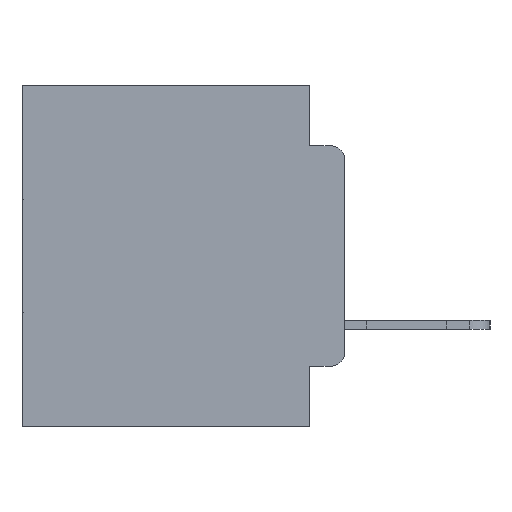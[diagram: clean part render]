
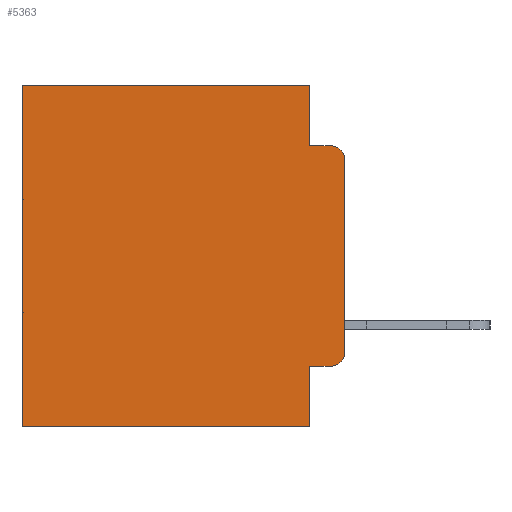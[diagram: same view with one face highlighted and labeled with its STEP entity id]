
A CAD part, left-side view. The second image highlights one B-rep face of the part: STEP entity #5363.
In plain terms, the highlighted planar face has unit normal (-1, 0, 0).
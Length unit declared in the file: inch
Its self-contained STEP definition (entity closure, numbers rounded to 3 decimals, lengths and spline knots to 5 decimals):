
#291 = EDGE_CURVE ( 'NONE', #7167, #15335, #7484, .T. ) ;
#449 = VERTEX_POINT ( 'NONE', #22604 ) ;
#1073 = VERTEX_POINT ( 'NONE', #19541 ) ;
#1476 = VERTEX_POINT ( 'NONE', #2860 ) ;
#1525 = DIRECTION ( 'NONE',  ( -1., 0., 0. ) ) ;
#1810 = ORIENTED_EDGE ( 'NONE', *, *, #14209, .T. ) ;
#1933 = VECTOR ( 'NONE', #9088, 39.37008 ) ;
#2264 = CARTESIAN_POINT ( 'NONE',  ( 0.298, 0.051, 0. ) ) ;
#2412 = ORIENTED_EDGE ( 'NONE', *, *, #7960, .T. ) ;
#2860 = CARTESIAN_POINT ( 'NONE',  ( 0.298, 0.473, -0.5 ) ) ;
#3824 = VERTEX_POINT ( 'NONE', #19217 ) ;
#3989 = CARTESIAN_POINT ( 'NONE',  ( 0.298, 0., 0. ) ) ;
#4005 = DIRECTION ( 'NONE',  ( 0., -1., 0. ) ) ;
#4414 = CARTESIAN_POINT ( 'NONE',  ( 0.298, 0., -0.5 ) ) ;
#4771 = FACE_OUTER_BOUND ( 'NONE', #26097, .T. ) ;
#5363 = ADVANCED_FACE ( 'NONE', ( #4771 ), #12246, .F. ) ;
#6403 = EDGE_CURVE ( 'NONE', #25711, #7167, #6469, .T. ) ;
#6469 = LINE ( 'NONE', #2264, #18177 ) ;
#7167 = VERTEX_POINT ( 'NONE', #20082 ) ;
#7484 = LINE ( 'NONE', #11281, #19053 ) ;
#7605 = VERTEX_POINT ( 'NONE', #22730 ) ;
#7831 = DIRECTION ( 'NONE',  ( 0., 0., -1. ) ) ;
#7960 = EDGE_CURVE ( 'NONE', #3824, #15335, #20650, .T. ) ;
#8324 = ORIENTED_EDGE ( 'NONE', *, *, #10698, .T. ) ;
#8485 = EDGE_CURVE ( 'NONE', #1073, #1476, #8627, .T. ) ;
#8627 = LINE ( 'NONE', #4414, #1933 ) ;
#8784 = VERTEX_POINT ( 'NONE', #15536 ) ;
#8816 = ORIENTED_EDGE ( 'NONE', *, *, #9880, .T. ) ;
#9088 = DIRECTION ( 'NONE',  ( 0., 1., 0. ) ) ;
#9880 = EDGE_CURVE ( 'NONE', #25711, #8784, #24725, .T. ) ;
#10514 = DIRECTION ( 'NONE',  ( 0., 1., 0. ) ) ;
#10698 = EDGE_CURVE ( 'NONE', #8784, #1476, #17287, .T. ) ;
#11136 = AXIS2_PLACEMENT_3D ( 'NONE', #26998, #1525, #18008 ) ;
#11281 = CARTESIAN_POINT ( 'NONE',  ( 0.298, 0.051, -0.0885 ) ) ;
#11382 = CARTESIAN_POINT ( 'NONE',  ( 0.298, 0.051, 0. ) ) ;
#11774 = ORIENTED_EDGE ( 'NONE', *, *, #6403, .F. ) ;
#11890 = VECTOR ( 'NONE', #7831, 39.37008 ) ;
#12166 = VECTOR ( 'NONE', #25401, 39.37008 ) ;
#12246 = PLANE ( 'NONE',  #12442 ) ;
#12442 = AXIS2_PLACEMENT_3D ( 'NONE', #13769, #15332, #23437 ) ;
#13073 = VECTOR ( 'NONE', #10514, 39.37008 ) ;
#13224 = DIRECTION ( 'NONE',  ( 0., 0., -1. ) ) ;
#13307 = LINE ( 'NONE', #29757, #24258 ) ;
#13460 = DIRECTION ( 'NONE',  ( 0., -1., 0. ) ) ;
#13769 = CARTESIAN_POINT ( 'NONE',  ( 0.298, 0., 0. ) ) ;
#13771 = DIRECTION ( 'NONE',  ( 0., 0., -1. ) ) ;
#14209 = EDGE_CURVE ( 'NONE', #449, #29352, #13307, .T. ) ;
#14313 = ORIENTED_EDGE ( 'NONE', *, *, #23508, .F. ) ;
#15332 = DIRECTION ( 'NONE',  ( 1., 0., 0. ) ) ;
#15335 = VERTEX_POINT ( 'NONE', #17015 ) ;
#15450 = ORIENTED_EDGE ( 'NONE', *, *, #291, .F. ) ;
#15484 = ORIENTED_EDGE ( 'NONE', *, *, #28410, .F. ) ;
#15513 = CARTESIAN_POINT ( 'NONE',  ( 0.298, 0.051, 0. ) ) ;
#15536 = CARTESIAN_POINT ( 'NONE',  ( 0.298, 0.473, 0. ) ) ;
#15918 = CARTESIAN_POINT ( 'NONE',  ( 0.298, 0.02, -0.1085 ) ) ;
#16271 = DIRECTION ( 'NONE',  ( 0., 0., -1. ) ) ;
#17015 = CARTESIAN_POINT ( 'NONE',  ( 0.298, 0.02, -0.0885 ) ) ;
#17287 = LINE ( 'NONE', #19872, #11890 ) ;
#18008 = DIRECTION ( 'NONE',  ( 0., 0., -1. ) ) ;
#18177 = VECTOR ( 'NONE', #16271, 39.37008 ) ;
#18669 = CARTESIAN_POINT ( 'NONE',  ( 0.298, 0.02, -0.4115 ) ) ;
#18683 = ORIENTED_EDGE ( 'NONE', *, *, #29575, .T. ) ;
#19053 = VECTOR ( 'NONE', #13460, 39.37008 ) ;
#19217 = CARTESIAN_POINT ( 'NONE',  ( 0.298, 0., -0.1085 ) ) ;
#19541 = CARTESIAN_POINT ( 'NONE',  ( 0.298, 0.051, -0.5 ) ) ;
#19795 = ORIENTED_EDGE ( 'NONE', *, *, #8485, .F. ) ;
#19872 = CARTESIAN_POINT ( 'NONE',  ( 0.298, 0.473, 0. ) ) ;
#20082 = CARTESIAN_POINT ( 'NONE',  ( 0.298, 0.051, -0.0885 ) ) ;
#20650 = CIRCLE ( 'NONE', #24309, 0.02 ) ;
#22604 = CARTESIAN_POINT ( 'NONE',  ( 0.298, 0.051, -0.4115 ) ) ;
#22730 = CARTESIAN_POINT ( 'NONE',  ( 0.298, 0., -0.3915 ) ) ;
#23437 = DIRECTION ( 'NONE',  ( 0., 0., -1. ) ) ;
#23508 = EDGE_CURVE ( 'NONE', #449, #1073, #24585, .T. ) ;
#23892 = VECTOR ( 'NONE', #13224, 39.37008 ) ;
#24258 = VECTOR ( 'NONE', #4005, 39.37008 ) ;
#24309 = AXIS2_PLACEMENT_3D ( 'NONE', #15918, #28979, #13771 ) ;
#24585 = LINE ( 'NONE', #11382, #23892 ) ;
#24590 = LINE ( 'NONE', #3989, #12166 ) ;
#24725 = LINE ( 'NONE', #24901, #13073 ) ;
#24901 = CARTESIAN_POINT ( 'NONE',  ( 0.298, 0., 0. ) ) ;
#25401 = DIRECTION ( 'NONE',  ( 0., 0., -1. ) ) ;
#25711 = VERTEX_POINT ( 'NONE', #15513 ) ;
#26097 = EDGE_LOOP ( 'NONE', ( #15484, #2412, #15450, #11774, #8816, #8324, #19795, #14313, #1810, #18683 ) ) ;
#26998 = CARTESIAN_POINT ( 'NONE',  ( 0.298, 0.02, -0.3915 ) ) ;
#28410 = EDGE_CURVE ( 'NONE', #3824, #7605, #24590, .T. ) ;
#28979 = DIRECTION ( 'NONE',  ( -1., 0., 0. ) ) ;
#29352 = VERTEX_POINT ( 'NONE', #18669 ) ;
#29490 = CIRCLE ( 'NONE', #11136, 0.02 ) ;
#29575 = EDGE_CURVE ( 'NONE', #29352, #7605, #29490, .T. ) ;
#29757 = CARTESIAN_POINT ( 'NONE',  ( 0.298, 0.051, -0.4115 ) ) ;
